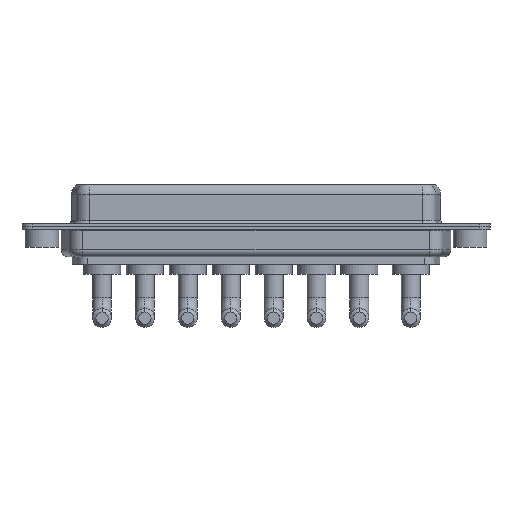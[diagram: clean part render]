
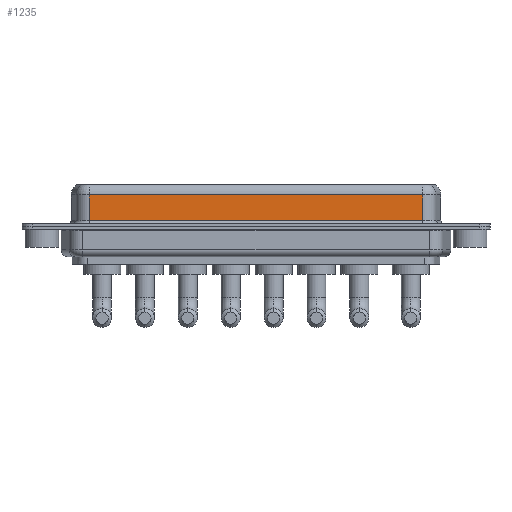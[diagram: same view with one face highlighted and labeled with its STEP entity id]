
A CAD part, front view. The second image highlights one B-rep face of the part: STEP entity #1235.
In plain terms, the highlighted planar face has unit normal (0, -1, 0).
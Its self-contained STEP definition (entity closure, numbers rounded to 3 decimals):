
#275 = EDGE_LOOP ( 'NONE', ( #351, #6389, #10474, #1621 ) ) ;
#351 = ORIENTED_EDGE ( 'NONE', *, *, #13229, .F. ) ;
#892 = DIRECTION ( 'NONE',  ( 0., 0., -1. ) ) ;
#1215 = DIRECTION ( 'NONE',  ( 0., 0., 1. ) ) ;
#1235 = ADVANCED_FACE ( 'NONE', ( #5115 ), #2096, .F. ) ;
#1585 = CARTESIAN_POINT ( 'NONE',  ( 56.462, -3.95, 0.9 ) ) ;
#1621 = ORIENTED_EDGE ( 'NONE', *, *, #3826, .T. ) ;
#2037 = DIRECTION ( 'NONE',  ( 0., 1., 0. ) ) ;
#2096 = PLANE ( 'NONE',  #11631 ) ;
#2622 = VECTOR ( 'NONE', #892, 1000. ) ;
#2796 = DIRECTION ( 'NONE',  ( -1., 0., 0. ) ) ;
#3614 = VERTEX_POINT ( 'NONE', #10056 ) ;
#3826 = EDGE_CURVE ( 'NONE', #12844, #12237, #13237, .T. ) ;
#4368 = DIRECTION ( 'NONE',  ( 0., 0., -1. ) ) ;
#4641 = CARTESIAN_POINT ( 'NONE',  ( 7.038, -3.95, 4.65 ) ) ;
#4912 = VECTOR ( 'NONE', #7150, 1000. ) ;
#5115 = FACE_OUTER_BOUND ( 'NONE', #275, .T. ) ;
#5246 = CARTESIAN_POINT ( 'NONE',  ( 56.462, -3.95, 0.9 ) ) ;
#5369 = CARTESIAN_POINT ( 'NONE',  ( 7.038, -3.95, 6.4 ) ) ;
#6258 = CARTESIAN_POINT ( 'NONE',  ( 56.462, -3.95, 6.4 ) ) ;
#6389 = ORIENTED_EDGE ( 'NONE', *, *, #8394, .T. ) ;
#7150 = DIRECTION ( 'NONE',  ( 1., 0., 0. ) ) ;
#7666 = LINE ( 'NONE', #5369, #9505 ) ;
#7939 = CARTESIAN_POINT ( 'NONE',  ( 56.462, -3.95, 4.65 ) ) ;
#8394 = EDGE_CURVE ( 'NONE', #3614, #11693, #13067, .T. ) ;
#9278 = VECTOR ( 'NONE', #2796, 1000. ) ;
#9300 = CARTESIAN_POINT ( 'NONE',  ( 56.462, -3.95, 6.4 ) ) ;
#9347 = EDGE_CURVE ( 'NONE', #11693, #12844, #7666, .T. ) ;
#9505 = VECTOR ( 'NONE', #4368, 1000. ) ;
#10056 = CARTESIAN_POINT ( 'NONE',  ( 56.462, -3.95, 4.65 ) ) ;
#10474 = ORIENTED_EDGE ( 'NONE', *, *, #9347, .T. ) ;
#11631 = AXIS2_PLACEMENT_3D ( 'NONE', #6258, #2037, #1215 ) ;
#11693 = VERTEX_POINT ( 'NONE', #4641 ) ;
#12237 = VERTEX_POINT ( 'NONE', #1585 ) ;
#12282 = LINE ( 'NONE', #9300, #2622 ) ;
#12844 = VERTEX_POINT ( 'NONE', #13309 ) ;
#13067 = LINE ( 'NONE', #7939, #9278 ) ;
#13229 = EDGE_CURVE ( 'NONE', #3614, #12237, #12282, .T. ) ;
#13237 = LINE ( 'NONE', #5246, #4912 ) ;
#13309 = CARTESIAN_POINT ( 'NONE',  ( 7.038, -3.95, 0.9 ) ) ;
